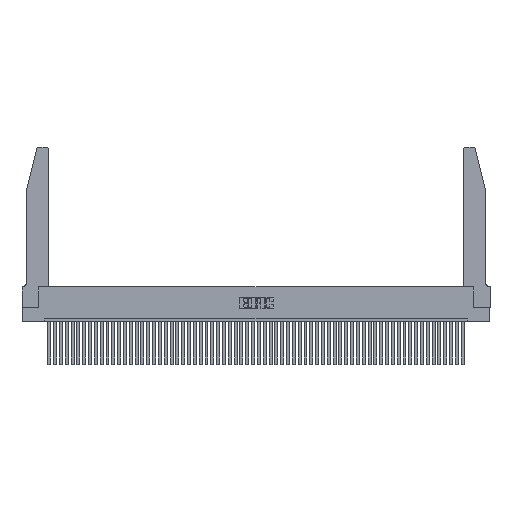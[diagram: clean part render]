
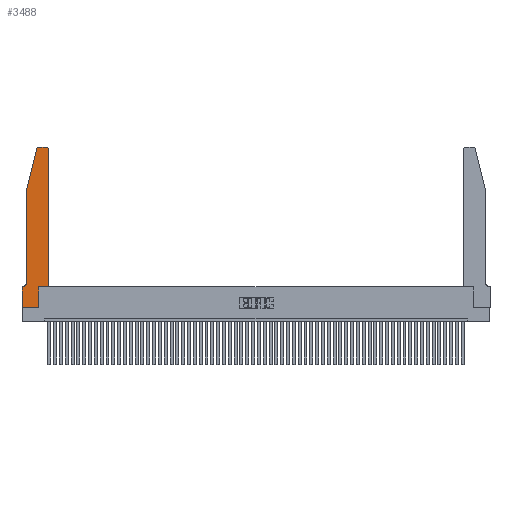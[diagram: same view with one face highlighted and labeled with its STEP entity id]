
A CAD part, top view. The second image highlights one B-rep face of the part: STEP entity #3488.
In plain terms, the highlighted planar face has unit normal (0, 0, 1).
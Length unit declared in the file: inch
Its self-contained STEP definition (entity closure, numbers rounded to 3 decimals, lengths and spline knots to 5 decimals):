
#2817 = LINE ( 'NONE', #28942, #22576 ) ;
#3488 = ADVANCED_FACE ( 'NONE', ( #11699 ), #11681, .T. ) ;
#3529 = EDGE_CURVE ( 'NONE', #45875, #38772, #32230, .T. ) ;
#3532 = LINE ( 'NONE', #16543, #28674 ) ;
#3754 = DIRECTION ( 'NONE',  ( 0., 1., 0. ) ) ;
#4990 = VECTOR ( 'NONE', #13529, 39.37008 ) ;
#5774 = EDGE_CURVE ( 'NONE', #23832, #33016, #7300, .T. ) ;
#6003 = CARTESIAN_POINT ( 'NONE',  ( 0.0755, 2., 0.37 ) ) ;
#6402 = CARTESIAN_POINT ( 'NONE',  ( 0.25487, 2.72718, 0.37 ) ) ;
#6681 = EDGE_CURVE ( 'NONE', #38772, #20586, #48099, .T. ) ;
#7300 = CIRCLE ( 'NONE', #18629, 0.03 ) ;
#7883 = CARTESIAN_POINT ( 'NONE',  ( 0., 0.35, 0.37 ) ) ;
#8030 = DIRECTION ( 'NONE',  ( 1., 0., 0. ) ) ;
#8206 = CARTESIAN_POINT ( 'NONE',  ( 0.2865, 0.35, 0.37 ) ) ;
#9182 = DIRECTION ( 'NONE',  ( -1., 0., 0. ) ) ;
#10391 = VECTOR ( 'NONE', #46020, 39.37008 ) ;
#11183 = AXIS2_PLACEMENT_3D ( 'NONE', #37200, #41658, #12239 ) ;
#11681 = PLANE ( 'NONE',  #36640 ) ;
#11699 = FACE_OUTER_BOUND ( 'NONE', #36695, .T. ) ;
#11943 = LINE ( 'NONE', #19024, #45010 ) ;
#12239 = DIRECTION ( 'NONE',  ( 1., 0., 0. ) ) ;
#13529 = DIRECTION ( 'NONE',  ( 0., -1., 0. ) ) ;
#15106 = CIRCLE ( 'NONE', #41551, 0.07 ) ;
#16217 = ORIENTED_EDGE ( 'NONE', *, *, #3529, .T. ) ;
#16282 = LINE ( 'NONE', #6003, #4990 ) ;
#16543 = CARTESIAN_POINT ( 'NONE',  ( 0.0755, 0.35, 0.37 ) ) ;
#16606 = DIRECTION ( 'NONE',  ( 1., 0., 0. ) ) ;
#17052 = LINE ( 'NONE', #19027, #10391 ) ;
#17561 = VERTEX_POINT ( 'NONE', #44819 ) ;
#18091 = CARTESIAN_POINT ( 'NONE',  ( 0.4505, 2.72, 0.37 ) ) ;
#18114 = CARTESIAN_POINT ( 'NONE',  ( 0.4205, 2.72, 0.37 ) ) ;
#18491 = DIRECTION ( 'NONE',  ( 0., 0., 1. ) ) ;
#18523 = CARTESIAN_POINT ( 'NONE',  ( 0.284, 2.75, 0.37 ) ) ;
#18629 = AXIS2_PLACEMENT_3D ( 'NONE', #18114, #18491, #23106 ) ;
#18917 = DIRECTION ( 'NONE',  ( 0., 0., -1. ) ) ;
#19024 = CARTESIAN_POINT ( 'NONE',  ( 0.0755, 2., 0.37 ) ) ;
#19027 = CARTESIAN_POINT ( 'NONE',  ( 0., 0., 0.37 ) ) ;
#19830 = VERTEX_POINT ( 'NONE', #18523 ) ;
#20572 = DIRECTION ( 'NONE',  ( 1., 0., 0. ) ) ;
#20586 = VERTEX_POINT ( 'NONE', #33645 ) ;
#20660 = EDGE_CURVE ( 'NONE', #42283, #52096, #3532, .T. ) ;
#20766 = LINE ( 'NONE', #22282, #34537 ) ;
#22282 = CARTESIAN_POINT ( 'NONE',  ( 0.2605, 2.75, 0.37 ) ) ;
#22411 = VERTEX_POINT ( 'NONE', #47621 ) ;
#22576 = VECTOR ( 'NONE', #8030, 39.37008 ) ;
#22985 = EDGE_CURVE ( 'NONE', #29322, #17561, #11943, .T. ) ;
#23106 = DIRECTION ( 'NONE',  ( 1., 0., 0. ) ) ;
#23226 = EDGE_CURVE ( 'NONE', #20586, #23832, #48922, .T. ) ;
#23722 = VECTOR ( 'NONE', #16606, 39.37008 ) ;
#23832 = VERTEX_POINT ( 'NONE', #18091 ) ;
#24829 = CARTESIAN_POINT ( 'NONE',  ( 0.4505, 0.35, 0.37 ) ) ;
#26893 = EDGE_CURVE ( 'NONE', #19830, #29322, #29305, .T. ) ;
#26900 = ORIENTED_EDGE ( 'NONE', *, *, #5774, .T. ) ;
#27207 = EDGE_CURVE ( 'NONE', #22411, #45875, #2817, .T. ) ;
#27808 = CARTESIAN_POINT ( 'NONE',  ( 0.0055, 0.42, 0.37 ) ) ;
#28674 = VECTOR ( 'NONE', #46463, 39.37008 ) ;
#28942 = CARTESIAN_POINT ( 'NONE',  ( 0., 0., 0.37 ) ) ;
#29305 = CIRCLE ( 'NONE', #11183, 0.03 ) ;
#29322 = VERTEX_POINT ( 'NONE', #6402 ) ;
#30523 = CARTESIAN_POINT ( 'NONE',  ( 0.0755, 0.42, 0.37 ) ) ;
#31468 = ORIENTED_EDGE ( 'NONE', *, *, #6681, .T. ) ;
#32230 = LINE ( 'NONE', #37196, #42170 ) ;
#33016 = VERTEX_POINT ( 'NONE', #51235 ) ;
#33645 = CARTESIAN_POINT ( 'NONE',  ( 0.4505, 0.35, 0.37 ) ) ;
#34255 = ORIENTED_EDGE ( 'NONE', *, *, #37717, .T. ) ;
#34537 = VECTOR ( 'NONE', #9182, 39.37008 ) ;
#35333 = CARTESIAN_POINT ( 'NONE',  ( 0.0055, 0.35, 0.37 ) ) ;
#35685 = DIRECTION ( 'NONE',  ( -1., 0., 0. ) ) ;
#36362 = VECTOR ( 'NONE', #45711, 39.37008 ) ;
#36640 = AXIS2_PLACEMENT_3D ( 'NONE', #54364, #37377, #20572 ) ;
#36695 = EDGE_LOOP ( 'NONE', ( #48516, #50260, #40583, #37938, #42652, #52548, #34255, #49943, #16217, #31468, #52636, #26900 ) ) ;
#37196 = CARTESIAN_POINT ( 'NONE',  ( 0.2865, 0.35, 0.37 ) ) ;
#37200 = CARTESIAN_POINT ( 'NONE',  ( 0.284, 2.72, 0.37 ) ) ;
#37377 = DIRECTION ( 'NONE',  ( 0., 0., 1. ) ) ;
#37717 = EDGE_CURVE ( 'NONE', #52096, #22411, #17052, .T. ) ;
#37938 = ORIENTED_EDGE ( 'NONE', *, *, #42333, .T. ) ;
#38772 = VERTEX_POINT ( 'NONE', #8206 ) ;
#40583 = ORIENTED_EDGE ( 'NONE', *, *, #22985, .T. ) ;
#41267 = CARTESIAN_POINT ( 'NONE',  ( 0.4505, 0.35, 0.37 ) ) ;
#41551 = AXIS2_PLACEMENT_3D ( 'NONE', #27808, #18917, #35685 ) ;
#41658 = DIRECTION ( 'NONE',  ( 0., 0., 1. ) ) ;
#42170 = VECTOR ( 'NONE', #3754, 39.37008 ) ;
#42283 = VERTEX_POINT ( 'NONE', #35333 ) ;
#42333 = EDGE_CURVE ( 'NONE', #17561, #52441, #16282, .T. ) ;
#42652 = ORIENTED_EDGE ( 'NONE', *, *, #49337, .T. ) ;
#43406 = EDGE_CURVE ( 'NONE', #33016, #19830, #20766, .T. ) ;
#44819 = CARTESIAN_POINT ( 'NONE',  ( 0.0755, 2., 0.37 ) ) ;
#45010 = VECTOR ( 'NONE', #48350, 39.37008 ) ;
#45711 = DIRECTION ( 'NONE',  ( 0., 1., 0. ) ) ;
#45875 = VERTEX_POINT ( 'NONE', #52832 ) ;
#46020 = DIRECTION ( 'NONE',  ( 0., -1., 0. ) ) ;
#46463 = DIRECTION ( 'NONE',  ( -1., 0., 0. ) ) ;
#47621 = CARTESIAN_POINT ( 'NONE',  ( 0., 0., 0.37 ) ) ;
#48099 = LINE ( 'NONE', #24829, #23722 ) ;
#48350 = DIRECTION ( 'NONE',  ( -0.239, -0.971, 0. ) ) ;
#48516 = ORIENTED_EDGE ( 'NONE', *, *, #43406, .T. ) ;
#48922 = LINE ( 'NONE', #41267, #36362 ) ;
#49337 = EDGE_CURVE ( 'NONE', #52441, #42283, #15106, .T. ) ;
#49943 = ORIENTED_EDGE ( 'NONE', *, *, #27207, .T. ) ;
#50260 = ORIENTED_EDGE ( 'NONE', *, *, #26893, .T. ) ;
#51235 = CARTESIAN_POINT ( 'NONE',  ( 0.4205, 2.75, 0.37 ) ) ;
#52096 = VERTEX_POINT ( 'NONE', #7883 ) ;
#52441 = VERTEX_POINT ( 'NONE', #30523 ) ;
#52548 = ORIENTED_EDGE ( 'NONE', *, *, #20660, .T. ) ;
#52636 = ORIENTED_EDGE ( 'NONE', *, *, #23226, .T. ) ;
#52832 = CARTESIAN_POINT ( 'NONE',  ( 0.2865, 0., 0.37 ) ) ;
#54364 = CARTESIAN_POINT ( 'NONE',  ( 0., 0.35, 0.37 ) ) ;
